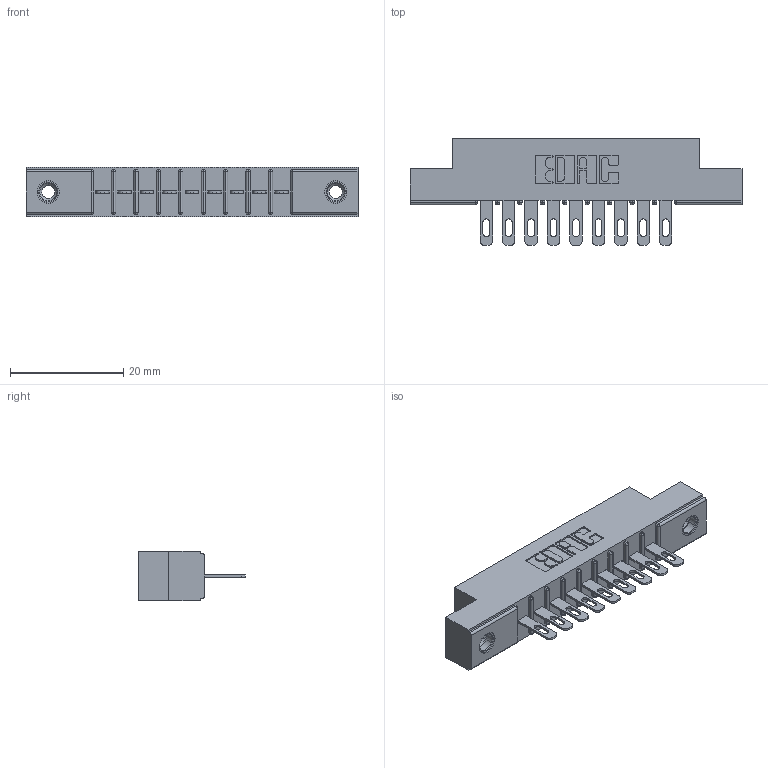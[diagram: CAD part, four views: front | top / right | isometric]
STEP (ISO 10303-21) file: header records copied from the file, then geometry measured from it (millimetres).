
FILE_DESCRIPTION (( 'STEP AP203' ), '1' );
FILE_NAME ('316-009-500-108.STEP', '2018-07-30T23:57:47', ( '' ), ( '' ), 'SwSTEP 2.0', 'SolidWorks 2016', '' );
FILE_SCHEMA (( 'CONFIG_CONTROL_DESIGN' ));
Length unit declared in the file: inch
Products named in the file (4): 306 Part_.156 Dia; 306-290-001_100; 345-250-001_345-250-003-102; 316-009-500-108
Assembly tree (12 placements, depth 2):
  316-009-500-108
    306 Part_.156 Dia
    306-290-001_100  x9
    345-250-001_345-250-003-102  x2
Bounding box: 58.67 x 18.87 x 8.71 mm (x, y, z)
Volume: 3981.9 mm3; surface area: 5636.3 mm2
Topology: 12 solids, 12 shells, 860 faces, 2387 edges, 1534 vertices
Faces by surface type: plane 550, cylinder 258, sphere 36, cone 12, torus 4
Entity records: 14017 total; most frequent: CARTESIAN_POINT 2329, DIRECTION 2309, ORIENTED_EDGE 2298, EDGE_CURVE 1149, VECTOR 877, LINE 877, VERTEX_POINT 736, AXIS2_PLACEMENT_3D 716
